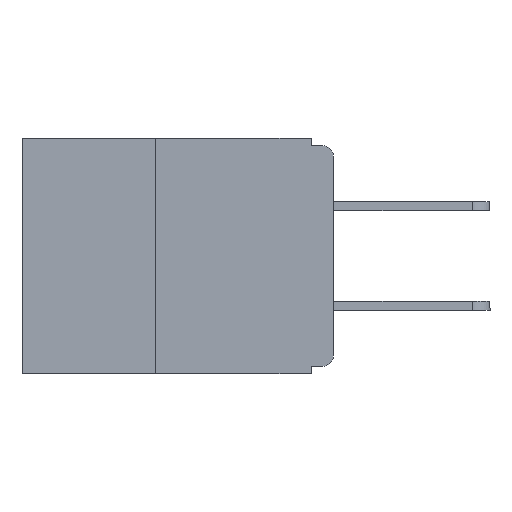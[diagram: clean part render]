
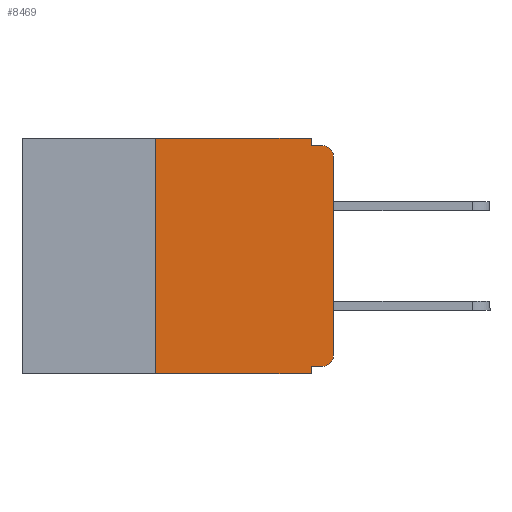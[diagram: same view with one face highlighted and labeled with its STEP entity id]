
A CAD part, left-side view. The second image highlights one B-rep face of the part: STEP entity #8469.
In plain terms, the highlighted planar face has unit normal (-1, 0, 0).
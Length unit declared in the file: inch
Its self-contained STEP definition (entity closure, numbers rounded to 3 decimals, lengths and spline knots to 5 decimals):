
#779 = LINE ( 'NONE', #30064, #35013 ) ;
#1291 = EDGE_LOOP ( 'NONE', ( #21030, #24289, #24606, #16003, #18064, #21203, #3448, #12038, #11423, #20975 ) ) ;
#1409 = VECTOR ( 'NONE', #4539, 39.37008 ) ;
#1960 = DIRECTION ( 'NONE',  ( 1., 0., 0. ) ) ;
#2623 = DIRECTION ( 'NONE',  ( 0., 0., -1. ) ) ;
#3448 = ORIENTED_EDGE ( 'NONE', *, *, #14015, .T. ) ;
#3486 = LINE ( 'NONE', #32105, #22355 ) ;
#3959 = VERTEX_POINT ( 'NONE', #19755 ) ;
#4045 = LINE ( 'NONE', #23548, #32660 ) ;
#4259 = CARTESIAN_POINT ( 'NONE',  ( 0., 0.25, -0.33 ) ) ;
#4539 = DIRECTION ( 'NONE',  ( 0., 0., -1. ) ) ;
#4733 = VERTEX_POINT ( 'NONE', #30888 ) ;
#4932 = CARTESIAN_POINT ( 'NONE',  ( 0., 0., -0.025 ) ) ;
#5279 = VERTEX_POINT ( 'NONE', #28252 ) ;
#5998 = DIRECTION ( 'NONE',  ( -1., 0., 0. ) ) ;
#6097 = EDGE_CURVE ( 'NONE', #23942, #4733, #4045, .T. ) ;
#6175 = VECTOR ( 'NONE', #16296, 39.37008 ) ;
#6643 = VERTEX_POINT ( 'NONE', #31723 ) ;
#6840 = DIRECTION ( 'NONE',  ( 0., 0., -1. ) ) ;
#7107 = DIRECTION ( 'NONE',  ( 0., 0., 1. ) ) ;
#8469 = ADVANCED_FACE ( 'NONE', ( #28076 ), #24235, .F. ) ;
#8891 = EDGE_CURVE ( 'NONE', #35810, #23942, #14269, .T. ) ;
#8976 = LINE ( 'NONE', #18587, #1409 ) ;
#9095 = EDGE_CURVE ( 'NONE', #3959, #6643, #8976, .T. ) ;
#9217 = CARTESIAN_POINT ( 'NONE',  ( 0., 0.25, -0.33 ) ) ;
#9505 = DIRECTION ( 'NONE',  ( 0., -1., 0. ) ) ;
#9627 = CARTESIAN_POINT ( 'NONE',  ( 0., 0., 0. ) ) ;
#10201 = VERTEX_POINT ( 'NONE', #29376 ) ;
#11423 = ORIENTED_EDGE ( 'NONE', *, *, #27840, .F. ) ;
#12038 = ORIENTED_EDGE ( 'NONE', *, *, #9095, .F. ) ;
#12098 = AXIS2_PLACEMENT_3D ( 'NONE', #18879, #1960, #21636 ) ;
#12618 = EDGE_CURVE ( 'NONE', #4733, #10201, #13698, .T. ) ;
#12871 = DIRECTION ( 'NONE',  ( 0., 1., 0. ) ) ;
#13587 = LINE ( 'NONE', #9627, #14470 ) ;
#13698 = LINE ( 'NONE', #32635, #6175 ) ;
#14015 = EDGE_CURVE ( 'NONE', #24510, #6643, #779, .T. ) ;
#14269 = LINE ( 'NONE', #20626, #35181 ) ;
#14470 = VECTOR ( 'NONE', #28982, 39.37008 ) ;
#15018 = CARTESIAN_POINT ( 'NONE',  ( 0., 0.031, 0. ) ) ;
#15696 = CIRCLE ( 'NONE', #24387, 0.015 ) ;
#16003 = ORIENTED_EDGE ( 'NONE', *, *, #6097, .F. ) ;
#16241 = EDGE_CURVE ( 'NONE', #30039, #10201, #15696, .T. ) ;
#16296 = DIRECTION ( 'NONE',  ( 0., -1., 0. ) ) ;
#17026 = EDGE_CURVE ( 'NONE', #24510, #35810, #28074, .T. ) ;
#18064 = ORIENTED_EDGE ( 'NONE', *, *, #8891, .F. ) ;
#18092 = AXIS2_PLACEMENT_3D ( 'NONE', #35699, #19507, #2623 ) ;
#18587 = CARTESIAN_POINT ( 'NONE',  ( 0., 0.031, -0.33 ) ) ;
#18879 = CARTESIAN_POINT ( 'NONE',  ( 0., 0.437, 0. ) ) ;
#19507 = DIRECTION ( 'NONE',  ( -1., 0., 0. ) ) ;
#19755 = CARTESIAN_POINT ( 'NONE',  ( 0., 0.031, -0.32 ) ) ;
#19987 = VECTOR ( 'NONE', #7107, 39.37008 ) ;
#20626 = CARTESIAN_POINT ( 'NONE',  ( 0., 0.437, 0. ) ) ;
#20975 = ORIENTED_EDGE ( 'NONE', *, *, #22094, .T. ) ;
#21030 = ORIENTED_EDGE ( 'NONE', *, *, #34409, .T. ) ;
#21203 = ORIENTED_EDGE ( 'NONE', *, *, #17026, .F. ) ;
#21636 = DIRECTION ( 'NONE',  ( 0., 0., -1. ) ) ;
#21981 = DIRECTION ( 'NONE',  ( 0., -1., 0. ) ) ;
#22094 = EDGE_CURVE ( 'NONE', #25368, #5279, #35279, .T. ) ;
#22355 = VECTOR ( 'NONE', #12871, 39.37008 ) ;
#22742 = CARTESIAN_POINT ( 'NONE',  ( 0., 0.015, -0.025 ) ) ;
#23548 = CARTESIAN_POINT ( 'NONE',  ( 0., 0.031, 0. ) ) ;
#23942 = VERTEX_POINT ( 'NONE', #15018 ) ;
#24212 = CARTESIAN_POINT ( 'NONE',  ( 0., 0.015, -0.32 ) ) ;
#24235 = PLANE ( 'NONE',  #12098 ) ;
#24289 = ORIENTED_EDGE ( 'NONE', *, *, #16241, .T. ) ;
#24387 = AXIS2_PLACEMENT_3D ( 'NONE', #22742, #5998, #25474 ) ;
#24510 = VERTEX_POINT ( 'NONE', #9217 ) ;
#24606 = ORIENTED_EDGE ( 'NONE', *, *, #12618, .F. ) ;
#25368 = VERTEX_POINT ( 'NONE', #24212 ) ;
#25474 = DIRECTION ( 'NONE',  ( 0., 0., -1. ) ) ;
#26602 = CARTESIAN_POINT ( 'NONE',  ( 0., 0.25, 0. ) ) ;
#27840 = EDGE_CURVE ( 'NONE', #25368, #3959, #3486, .T. ) ;
#28074 = LINE ( 'NONE', #4259, #19987 ) ;
#28076 = FACE_OUTER_BOUND ( 'NONE', #1291, .T. ) ;
#28252 = CARTESIAN_POINT ( 'NONE',  ( 0., 0., -0.305 ) ) ;
#28982 = DIRECTION ( 'NONE',  ( 0., 0., 1. ) ) ;
#29376 = CARTESIAN_POINT ( 'NONE',  ( 0., 0.015, -0.01 ) ) ;
#30039 = VERTEX_POINT ( 'NONE', #4932 ) ;
#30064 = CARTESIAN_POINT ( 'NONE',  ( 0., 0.437, -0.33 ) ) ;
#30888 = CARTESIAN_POINT ( 'NONE',  ( 0., 0.031, -0.01 ) ) ;
#31723 = CARTESIAN_POINT ( 'NONE',  ( 0., 0.031, -0.33 ) ) ;
#32105 = CARTESIAN_POINT ( 'NONE',  ( 0., 0., -0.32 ) ) ;
#32635 = CARTESIAN_POINT ( 'NONE',  ( 0., 0., -0.01 ) ) ;
#32660 = VECTOR ( 'NONE', #6840, 39.37008 ) ;
#34409 = EDGE_CURVE ( 'NONE', #5279, #30039, #13587, .T. ) ;
#35013 = VECTOR ( 'NONE', #21981, 39.37008 ) ;
#35181 = VECTOR ( 'NONE', #9505, 39.37008 ) ;
#35279 = CIRCLE ( 'NONE', #18092, 0.015 ) ;
#35699 = CARTESIAN_POINT ( 'NONE',  ( 0., 0.015, -0.305 ) ) ;
#35810 = VERTEX_POINT ( 'NONE', #26602 ) ;
